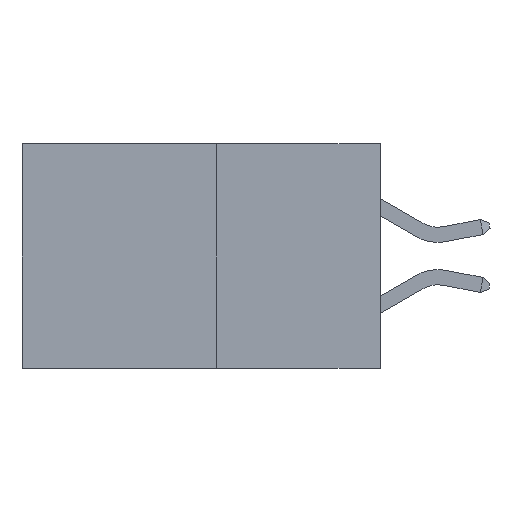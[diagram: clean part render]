
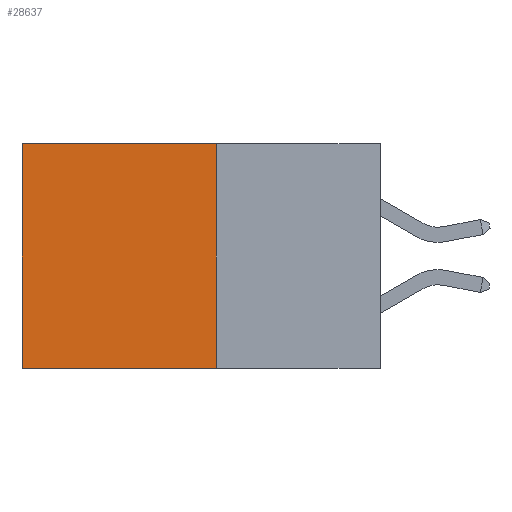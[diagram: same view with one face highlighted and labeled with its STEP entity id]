
A CAD part, left-side view. The second image highlights one B-rep face of the part: STEP entity #28637.
In plain terms, the highlighted planar face has unit normal (-1, 0, 0).
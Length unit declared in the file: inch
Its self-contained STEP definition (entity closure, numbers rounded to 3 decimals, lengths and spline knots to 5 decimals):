
#49 = ORIENTED_EDGE ( 'NONE', *, *, #15462, .F. ) ;
#1725 = ORIENTED_EDGE ( 'NONE', *, *, #5471, .F. ) ;
#3501 = PLANE ( 'NONE',  #13829 ) ;
#3609 = VERTEX_POINT ( 'NONE', #19652 ) ;
#5471 = EDGE_CURVE ( 'NONE', #21449, #13399, #6274, .T. ) ;
#5956 = DIRECTION ( 'NONE',  ( 0., 0., -1. ) ) ;
#6274 = LINE ( 'NONE', #21719, #11350 ) ;
#7642 = ORIENTED_EDGE ( 'NONE', *, *, #18290, .T. ) ;
#8018 = ORIENTED_EDGE ( 'NONE', *, *, #19105, .T. ) ;
#9813 = VERTEX_POINT ( 'NONE', #28237 ) ;
#9842 = FACE_OUTER_BOUND ( 'NONE', #23045, .T. ) ;
#10862 = CARTESIAN_POINT ( 'NONE',  ( 0.277, 0.27, -0.37 ) ) ;
#11319 = DIRECTION ( 'NONE',  ( 0., 0., -1. ) ) ;
#11350 = VECTOR ( 'NONE', #16836, 39.37008 ) ;
#11582 = VECTOR ( 'NONE', #21170, 39.37008 ) ;
#13040 = LINE ( 'NONE', #23626, #31116 ) ;
#13399 = VERTEX_POINT ( 'NONE', #18325 ) ;
#13829 = AXIS2_PLACEMENT_3D ( 'NONE', #10862, #20798, #5956 ) ;
#15462 = EDGE_CURVE ( 'NONE', #9813, #21449, #13040, .T. ) ;
#16836 = DIRECTION ( 'NONE',  ( 0., 1., 0. ) ) ;
#17004 = DIRECTION ( 'NONE',  ( 0., 1., 0. ) ) ;
#18290 = EDGE_CURVE ( 'NONE', #9813, #3609, #24032, .T. ) ;
#18325 = CARTESIAN_POINT ( 'NONE',  ( 0.277, 0.59, -0.37 ) ) ;
#18704 = CARTESIAN_POINT ( 'NONE',  ( 0.277, 0.59, -0.37 ) ) ;
#19105 = EDGE_CURVE ( 'NONE', #3609, #13399, #24730, .T. ) ;
#19652 = CARTESIAN_POINT ( 'NONE',  ( 0.277, 0.59, 0. ) ) ;
#20798 = DIRECTION ( 'NONE',  ( 1., 0., 0. ) ) ;
#21170 = DIRECTION ( 'NONE',  ( 0., 0., -1. ) ) ;
#21449 = VERTEX_POINT ( 'NONE', #27202 ) ;
#21719 = CARTESIAN_POINT ( 'NONE',  ( 0.277, 0.27, -0.37 ) ) ;
#23045 = EDGE_LOOP ( 'NONE', ( #8018, #1725, #49, #7642 ) ) ;
#23626 = CARTESIAN_POINT ( 'NONE',  ( 0.277, 0.27, -0.37 ) ) ;
#24032 = LINE ( 'NONE', #31739, #24824 ) ;
#24730 = LINE ( 'NONE', #18704, #11582 ) ;
#24824 = VECTOR ( 'NONE', #17004, 39.37008 ) ;
#27202 = CARTESIAN_POINT ( 'NONE',  ( 0.277, 0.27, -0.37 ) ) ;
#28237 = CARTESIAN_POINT ( 'NONE',  ( 0.277, 0.27, 0. ) ) ;
#28637 = ADVANCED_FACE ( 'NONE', ( #9842 ), #3501, .F. ) ;
#31116 = VECTOR ( 'NONE', #11319, 39.37008 ) ;
#31739 = CARTESIAN_POINT ( 'NONE',  ( 0.277, 0.27, 0. ) ) ;
